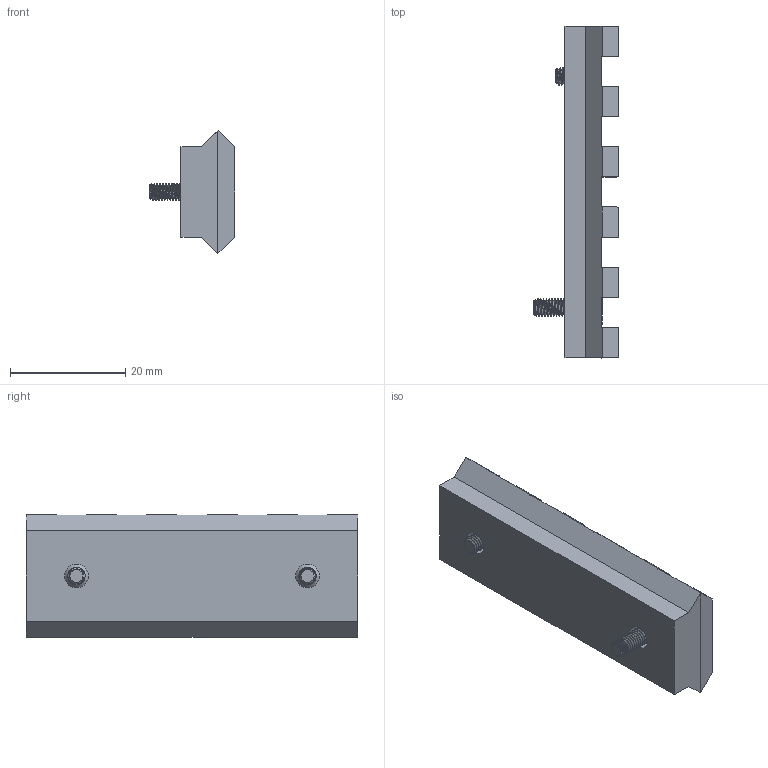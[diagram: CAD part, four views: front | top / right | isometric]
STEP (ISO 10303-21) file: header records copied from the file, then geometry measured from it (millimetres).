
FILE_DESCRIPTION(/* description */ (''),/* implementation_level */ '2;1');
FILE_NAME(/* name */ 'Picatinny Plates (Side).step',/* time_stamp */ '2023-01-02T15:48:39-05:00',/* author */ (''),/* organization */ (''),/* preprocessor_version */ 'ST-DEVELOPER v19.2',/* originating_system */ 'Autodesk Translation Framework v11.17.0.187',/* authorisation */ '');
FILE_SCHEMA (('AUTOMOTIVE_DESIGN { 1 0 10303 214 3 1 1 }'));
Length unit declared in the file: millimetre
Products named in the file (3): Picatinny Plates (Side); 91294A128; 91294A132
Assembly tree (2 placements, depth 2):
  Picatinny Plates (Side)
    91294A128
    91294A132
Bounding box: 14.82 x 57.56 x 21.21 mm (x, y, z)
Volume: 7826.2 mm3; surface area: 4422.5 mm2
Topology: 3 solids, 3 shells, 158 faces, 412 edges, 262 vertices
Faces by surface type: cylinder 74, plane 62, cone 18, bspline 4
Full cylindrical faces by diameter (mm): 2.35 x30, 3 x30, 4.1 x2, 6 x2
Entity records: 11236 total; most frequent: CARTESIAN_POINT 7585, ORIENTED_EDGE 824, DIRECTION 611, EDGE_CURVE 412, VERTEX_POINT 262, LINE 215, VECTOR 215, AXIS2_PLACEMENT_3D 198
